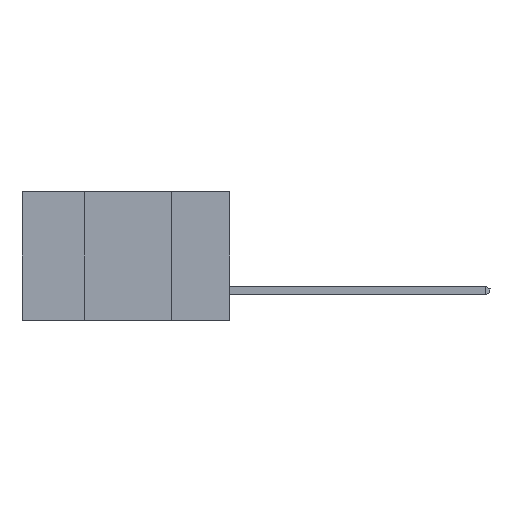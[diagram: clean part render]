
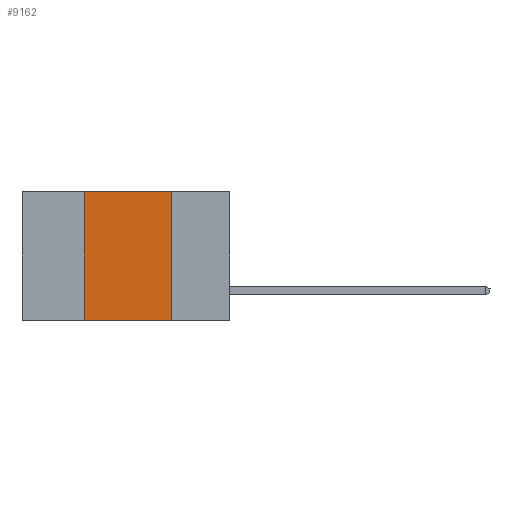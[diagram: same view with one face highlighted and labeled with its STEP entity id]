
A CAD part, left-side view. The second image highlights one B-rep face of the part: STEP entity #9162.
In plain terms, the highlighted planar face has unit normal (-1, 0, 0).
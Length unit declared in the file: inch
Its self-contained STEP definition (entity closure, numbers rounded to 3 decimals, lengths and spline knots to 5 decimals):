
#1928 = DIRECTION ( 'NONE',  ( 0., -1., 0. ) ) ;
#1935 = VERTEX_POINT ( 'NONE', #3987 ) ;
#2249 = CARTESIAN_POINT ( 'NONE',  ( 0., 0.6, -0.37 ) ) ;
#2698 = VECTOR ( 'NONE', #3663, 39.37008 ) ;
#3663 = DIRECTION ( 'NONE',  ( 0., 0., 1. ) ) ;
#3987 = CARTESIAN_POINT ( 'NONE',  ( 0., 0.17, -0.37 ) ) ;
#4980 = EDGE_CURVE ( 'NONE', #23283, #1935, #14618, .T. ) ;
#5072 = AXIS2_PLACEMENT_3D ( 'NONE', #7232, #11013, #14776 ) ;
#5437 = CARTESIAN_POINT ( 'NONE',  ( 0., 0.42, -0.37 ) ) ;
#6908 = CARTESIAN_POINT ( 'NONE',  ( 0., 0.17, 0. ) ) ;
#7232 = CARTESIAN_POINT ( 'NONE',  ( 0., 0.6, 0. ) ) ;
#9114 = PLANE ( 'NONE',  #5072 ) ;
#9162 = ADVANCED_FACE ( 'NONE', ( #11127 ), #9114, .F. ) ;
#9628 = EDGE_CURVE ( 'NONE', #14386, #1935, #9927, .T. ) ;
#9927 = LINE ( 'NONE', #2249, #18402 ) ;
#10429 = ORIENTED_EDGE ( 'NONE', *, *, #10632, .F. ) ;
#10632 = EDGE_CURVE ( 'NONE', #20674, #23283, #11496, .T. ) ;
#11013 = DIRECTION ( 'NONE',  ( 1., 0., 0. ) ) ;
#11088 = CARTESIAN_POINT ( 'NONE',  ( 0., 0.42, -0.37 ) ) ;
#11127 = FACE_OUTER_BOUND ( 'NONE', #11961, .T. ) ;
#11496 = LINE ( 'NONE', #19190, #21040 ) ;
#11961 = EDGE_LOOP ( 'NONE', ( #19931, #10429, #12176, #13692 ) ) ;
#12176 = ORIENTED_EDGE ( 'NONE', *, *, #13126, .F. ) ;
#12727 = DIRECTION ( 'NONE',  ( 0., 0., -1. ) ) ;
#13126 = EDGE_CURVE ( 'NONE', #14386, #20674, #20671, .T. ) ;
#13386 = VECTOR ( 'NONE', #12727, 39.37008 ) ;
#13692 = ORIENTED_EDGE ( 'NONE', *, *, #9628, .T. ) ;
#14386 = VERTEX_POINT ( 'NONE', #5437 ) ;
#14496 = CARTESIAN_POINT ( 'NONE',  ( 0., 0.17, -0.37 ) ) ;
#14618 = LINE ( 'NONE', #14496, #13386 ) ;
#14776 = DIRECTION ( 'NONE',  ( 0., 0., -1. ) ) ;
#17493 = DIRECTION ( 'NONE',  ( 0., -1., 0. ) ) ;
#18402 = VECTOR ( 'NONE', #17493, 39.37008 ) ;
#19190 = CARTESIAN_POINT ( 'NONE',  ( 0., 0.6, 0. ) ) ;
#19931 = ORIENTED_EDGE ( 'NONE', *, *, #4980, .F. ) ;
#20671 = LINE ( 'NONE', #11088, #2698 ) ;
#20674 = VERTEX_POINT ( 'NONE', #21249 ) ;
#21040 = VECTOR ( 'NONE', #1928, 39.37008 ) ;
#21249 = CARTESIAN_POINT ( 'NONE',  ( 0., 0.42, 0. ) ) ;
#23283 = VERTEX_POINT ( 'NONE', #6908 ) ;
